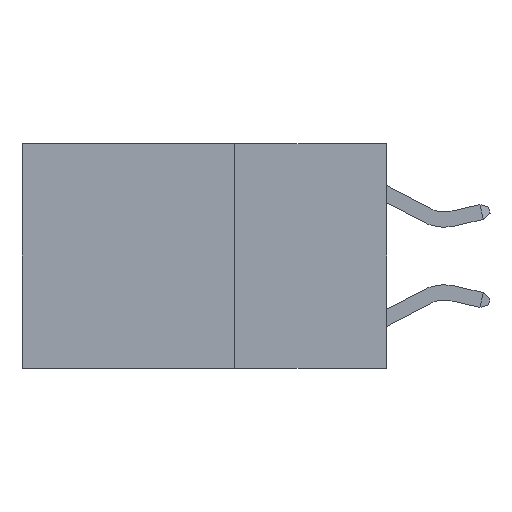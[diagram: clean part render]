
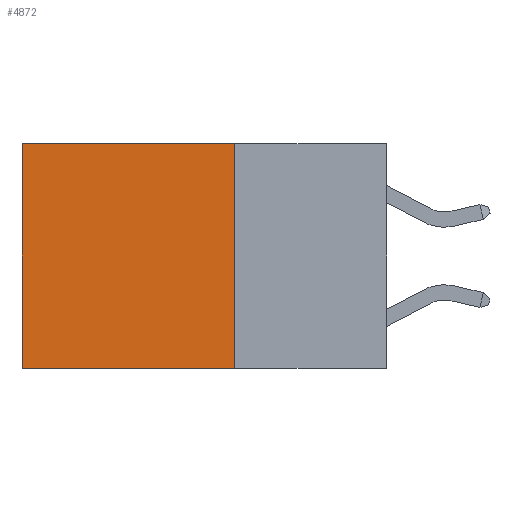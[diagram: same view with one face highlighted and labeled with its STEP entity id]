
A CAD part, left-side view. The second image highlights one B-rep face of the part: STEP entity #4872.
In plain terms, the highlighted planar face has unit normal (-1, 0, 0).
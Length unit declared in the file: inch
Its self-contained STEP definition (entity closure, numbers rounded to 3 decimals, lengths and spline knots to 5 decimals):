
#609 = EDGE_CURVE ( 'NONE', #7189, #2799, #3933, .T. ) ;
#844 = AXIS2_PLACEMENT_3D ( 'NONE', #1986, #9545, #2182 ) ;
#1487 = DIRECTION ( 'NONE',  ( 0., 1., 0. ) ) ;
#1687 = DIRECTION ( 'NONE',  ( 0., 0., -1. ) ) ;
#1767 = EDGE_CURVE ( 'NONE', #13271, #14391, #7530, .T. ) ;
#1789 = CARTESIAN_POINT ( 'NONE',  ( 0.2625, 0.6, 0. ) ) ;
#1886 = ORIENTED_EDGE ( 'NONE', *, *, #2976, .T. ) ;
#1986 = CARTESIAN_POINT ( 'NONE',  ( 0.2625, 0.25, 0. ) ) ;
#2182 = DIRECTION ( 'NONE',  ( 0., 0., -1. ) ) ;
#2630 = CARTESIAN_POINT ( 'NONE',  ( 0.2625, 0.6, 0. ) ) ;
#2751 = ORIENTED_EDGE ( 'NONE', *, *, #1767, .T. ) ;
#2771 = VECTOR ( 'NONE', #12226, 39.37008 ) ;
#2799 = VERTEX_POINT ( 'NONE', #6538 ) ;
#2976 = EDGE_CURVE ( 'NONE', #14391, #2799, #5369, .T. ) ;
#3042 = CARTESIAN_POINT ( 'NONE',  ( 0.2625, 0.25, 0. ) ) ;
#3933 = LINE ( 'NONE', #14508, #2771 ) ;
#3971 = CARTESIAN_POINT ( 'NONE',  ( 0.2625, 0.25, 0. ) ) ;
#4872 = ADVANCED_FACE ( 'NONE', ( #13583 ), #5669, .F. ) ;
#5369 = LINE ( 'NONE', #1789, #11157 ) ;
#5669 = PLANE ( 'NONE',  #844 ) ;
#6538 = CARTESIAN_POINT ( 'NONE',  ( 0.2625, 0.6, -0.37 ) ) ;
#7189 = VERTEX_POINT ( 'NONE', #9844 ) ;
#7530 = LINE ( 'NONE', #3971, #13685 ) ;
#8043 = LINE ( 'NONE', #14238, #13230 ) ;
#8874 = EDGE_LOOP ( 'NONE', ( #1886, #13788, #8951, #2751 ) ) ;
#8951 = ORIENTED_EDGE ( 'NONE', *, *, #14038, .F. ) ;
#9545 = DIRECTION ( 'NONE',  ( 1., 0., 0. ) ) ;
#9844 = CARTESIAN_POINT ( 'NONE',  ( 0.2625, 0.25, -0.37 ) ) ;
#11157 = VECTOR ( 'NONE', #1687, 39.37008 ) ;
#12226 = DIRECTION ( 'NONE',  ( 0., 1., 0. ) ) ;
#13230 = VECTOR ( 'NONE', #15523, 39.37008 ) ;
#13271 = VERTEX_POINT ( 'NONE', #3042 ) ;
#13583 = FACE_OUTER_BOUND ( 'NONE', #8874, .T. ) ;
#13685 = VECTOR ( 'NONE', #1487, 39.37008 ) ;
#13788 = ORIENTED_EDGE ( 'NONE', *, *, #609, .F. ) ;
#14038 = EDGE_CURVE ( 'NONE', #13271, #7189, #8043, .T. ) ;
#14238 = CARTESIAN_POINT ( 'NONE',  ( 0.2625, 0.25, 0. ) ) ;
#14391 = VERTEX_POINT ( 'NONE', #2630 ) ;
#14508 = CARTESIAN_POINT ( 'NONE',  ( 0.2625, 0.25, -0.37 ) ) ;
#15523 = DIRECTION ( 'NONE',  ( 0., 0., -1. ) ) ;
